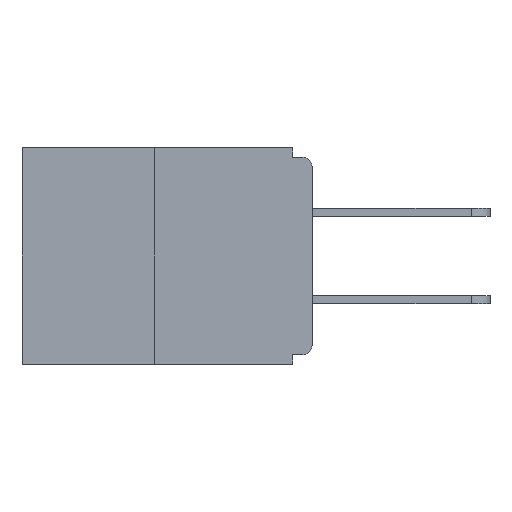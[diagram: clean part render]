
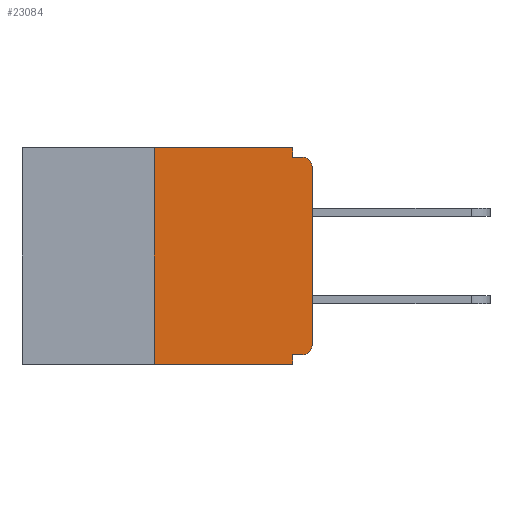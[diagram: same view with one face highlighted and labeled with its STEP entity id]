
A CAD part, left-side view. The second image highlights one B-rep face of the part: STEP entity #23084.
In plain terms, the highlighted planar face has unit normal (-1, 0, 0).
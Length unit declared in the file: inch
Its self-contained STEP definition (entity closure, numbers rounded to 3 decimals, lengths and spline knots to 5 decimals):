
#14 = CARTESIAN_POINT ( 'NONE',  ( 0., 0.25, 0. ) ) ;
#223 = VERTEX_POINT ( 'NONE', #14 ) ;
#683 = VECTOR ( 'NONE', #4021, 39.37008 ) ;
#705 = VERTEX_POINT ( 'NONE', #8047 ) ;
#884 = ORIENTED_EDGE ( 'NONE', *, *, #27078, .F. ) ;
#995 = CARTESIAN_POINT ( 'NONE',  ( 0., 0.031, 0. ) ) ;
#1084 = CARTESIAN_POINT ( 'NONE',  ( 0., 0.015, -0.313 ) ) ;
#1466 = CARTESIAN_POINT ( 'NONE',  ( 0., 0.46, -0.343 ) ) ;
#1543 = CARTESIAN_POINT ( 'NONE',  ( 0., 0., 0. ) ) ;
#2282 = CIRCLE ( 'NONE', #19178, 0.015 ) ;
#3132 = LINE ( 'NONE', #1466, #24437 ) ;
#3233 = AXIS2_PLACEMENT_3D ( 'NONE', #23963, #17832, #9172 ) ;
#3254 = DIRECTION ( 'NONE',  ( 0., 0., -1. ) ) ;
#3847 = DIRECTION ( 'NONE',  ( 0., 0., -1. ) ) ;
#4021 = DIRECTION ( 'NONE',  ( 0., -1., 0. ) ) ;
#4156 = EDGE_CURVE ( 'NONE', #12037, #20212, #2282, .T. ) ;
#5725 = CARTESIAN_POINT ( 'NONE',  ( 0., 0.031, -0.343 ) ) ;
#5853 = DIRECTION ( 'NONE',  ( 0., 0., -1. ) ) ;
#5941 = DIRECTION ( 'NONE',  ( -1., 0., 0. ) ) ;
#7267 = VECTOR ( 'NONE', #22827, 39.37008 ) ;
#7305 = EDGE_CURVE ( 'NONE', #23178, #17947, #3132, .T. ) ;
#7462 = EDGE_CURVE ( 'NONE', #23178, #223, #9154, .T. ) ;
#8047 = CARTESIAN_POINT ( 'NONE',  ( 0., 0.031, 0. ) ) ;
#8189 = EDGE_CURVE ( 'NONE', #223, #705, #14806, .T. ) ;
#8953 = FACE_OUTER_BOUND ( 'NONE', #9255, .T. ) ;
#9154 = LINE ( 'NONE', #19007, #21482 ) ;
#9172 = DIRECTION ( 'NONE',  ( 0., 0., -1. ) ) ;
#9255 = EDGE_LOOP ( 'NONE', ( #23186, #14437, #24560, #23714, #9546, #13525, #24306, #12957, #20741, #884 ) ) ;
#9546 = ORIENTED_EDGE ( 'NONE', *, *, #13307, .F. ) ;
#10112 = DIRECTION ( 'NONE',  ( -1., 0., 0. ) ) ;
#10360 = DIRECTION ( 'NONE',  ( 0., 0., 1. ) ) ;
#10860 = CARTESIAN_POINT ( 'NONE',  ( 0., 0.031, -0.343 ) ) ;
#11703 = VERTEX_POINT ( 'NONE', #21830 ) ;
#11711 = VERTEX_POINT ( 'NONE', #21926 ) ;
#12028 = LINE ( 'NONE', #14664, #17397 ) ;
#12037 = VERTEX_POINT ( 'NONE', #19627 ) ;
#12790 = EDGE_CURVE ( 'NONE', #11703, #20212, #23415, .T. ) ;
#12957 = ORIENTED_EDGE ( 'NONE', *, *, #4156, .T. ) ;
#13018 = VERTEX_POINT ( 'NONE', #24272 ) ;
#13307 = EDGE_CURVE ( 'NONE', #17330, #13018, #12028, .T. ) ;
#13525 = ORIENTED_EDGE ( 'NONE', *, *, #21266, .T. ) ;
#14437 = ORIENTED_EDGE ( 'NONE', *, *, #7462, .F. ) ;
#14664 = CARTESIAN_POINT ( 'NONE',  ( 0., 0., -0.328 ) ) ;
#14806 = LINE ( 'NONE', #20326, #15456 ) ;
#14988 = EDGE_CURVE ( 'NONE', #11711, #12037, #24568, .T. ) ;
#15284 = VECTOR ( 'NONE', #3847, 39.37008 ) ;
#15456 = VECTOR ( 'NONE', #22464, 39.37008 ) ;
#16483 = AXIS2_PLACEMENT_3D ( 'NONE', #1084, #10112, #3254 ) ;
#16875 = EDGE_CURVE ( 'NONE', #13018, #17947, #27540, .T. ) ;
#17330 = VERTEX_POINT ( 'NONE', #26928 ) ;
#17397 = VECTOR ( 'NONE', #18927, 39.37008 ) ;
#17832 = DIRECTION ( 'NONE',  ( 1., 0., 0. ) ) ;
#17947 = VERTEX_POINT ( 'NONE', #10860 ) ;
#18594 = CARTESIAN_POINT ( 'NONE',  ( 0., 0.015, -0.03 ) ) ;
#18754 = DIRECTION ( 'NONE',  ( 0., 0., -1. ) ) ;
#18927 = DIRECTION ( 'NONE',  ( 0., 1., 0. ) ) ;
#19007 = CARTESIAN_POINT ( 'NONE',  ( 0., 0.25, 0. ) ) ;
#19178 = AXIS2_PLACEMENT_3D ( 'NONE', #18594, #5941, #5853 ) ;
#19507 = VECTOR ( 'NONE', #18754, 39.37008 ) ;
#19627 = CARTESIAN_POINT ( 'NONE',  ( 0., 0., -0.03 ) ) ;
#20212 = VERTEX_POINT ( 'NONE', #24818 ) ;
#20322 = DIRECTION ( 'NONE',  ( 0., -1., 0. ) ) ;
#20326 = CARTESIAN_POINT ( 'NONE',  ( 0., 0.46, 0. ) ) ;
#20741 = ORIENTED_EDGE ( 'NONE', *, *, #12790, .F. ) ;
#21266 = EDGE_CURVE ( 'NONE', #17330, #11711, #22353, .T. ) ;
#21482 = VECTOR ( 'NONE', #10360, 39.37008 ) ;
#21737 = PLANE ( 'NONE',  #3233 ) ;
#21830 = CARTESIAN_POINT ( 'NONE',  ( 0., 0.031, -0.015 ) ) ;
#21926 = CARTESIAN_POINT ( 'NONE',  ( 0., 0., -0.313 ) ) ;
#22353 = CIRCLE ( 'NONE', #16483, 0.015 ) ;
#22464 = DIRECTION ( 'NONE',  ( 0., -1., 0. ) ) ;
#22827 = DIRECTION ( 'NONE',  ( 0., 0., 1. ) ) ;
#23084 = ADVANCED_FACE ( 'NONE', ( #8953 ), #21737, .F. ) ;
#23178 = VERTEX_POINT ( 'NONE', #24799 ) ;
#23186 = ORIENTED_EDGE ( 'NONE', *, *, #8189, .F. ) ;
#23415 = LINE ( 'NONE', #27427, #683 ) ;
#23714 = ORIENTED_EDGE ( 'NONE', *, *, #16875, .F. ) ;
#23963 = CARTESIAN_POINT ( 'NONE',  ( 0., 0.46, 0. ) ) ;
#24272 = CARTESIAN_POINT ( 'NONE',  ( 0., 0.031, -0.328 ) ) ;
#24306 = ORIENTED_EDGE ( 'NONE', *, *, #14988, .T. ) ;
#24437 = VECTOR ( 'NONE', #20322, 39.37008 ) ;
#24560 = ORIENTED_EDGE ( 'NONE', *, *, #7305, .T. ) ;
#24568 = LINE ( 'NONE', #1543, #7267 ) ;
#24799 = CARTESIAN_POINT ( 'NONE',  ( 0., 0.25, -0.343 ) ) ;
#24818 = CARTESIAN_POINT ( 'NONE',  ( 0., 0.015, -0.015 ) ) ;
#25960 = LINE ( 'NONE', #995, #15284 ) ;
#26928 = CARTESIAN_POINT ( 'NONE',  ( 0., 0.015, -0.328 ) ) ;
#27078 = EDGE_CURVE ( 'NONE', #705, #11703, #25960, .T. ) ;
#27427 = CARTESIAN_POINT ( 'NONE',  ( 0., 0., -0.015 ) ) ;
#27540 = LINE ( 'NONE', #5725, #19507 ) ;
